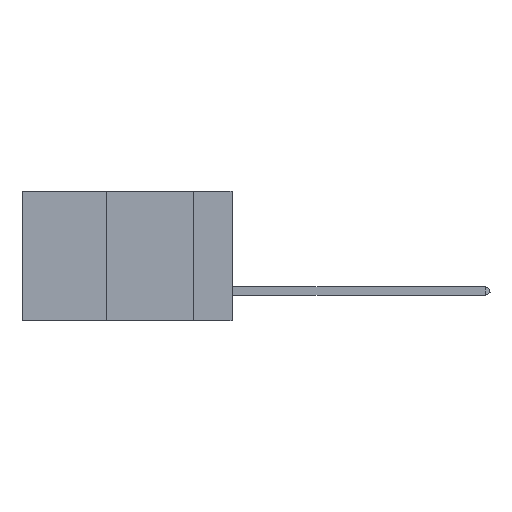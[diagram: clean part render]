
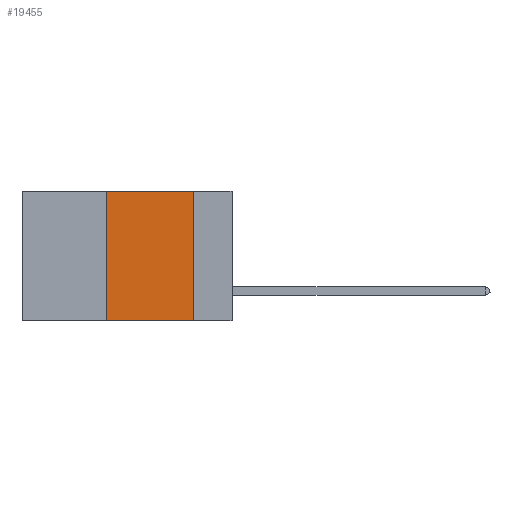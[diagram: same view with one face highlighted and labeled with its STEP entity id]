
A CAD part, left-side view. The second image highlights one B-rep face of the part: STEP entity #19455.
In plain terms, the highlighted planar face has unit normal (-1, 0, 0).
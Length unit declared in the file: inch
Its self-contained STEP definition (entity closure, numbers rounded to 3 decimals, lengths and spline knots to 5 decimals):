
#2512 = EDGE_LOOP ( 'NONE', ( #15538, #45953, #48157, #13108 ) ) ;
#3488 = LINE ( 'NONE', #41045, #7559 ) ;
#4142 = AXIS2_PLACEMENT_3D ( 'NONE', #28260, #43907, #5815 ) ;
#5815 = DIRECTION ( 'NONE',  ( 0., 0., -1. ) ) ;
#7559 = VECTOR ( 'NONE', #26187, 39.37008 ) ;
#9216 = CARTESIAN_POINT ( 'NONE',  ( 0., 0.6, -0.37 ) ) ;
#12147 = LINE ( 'NONE', #9216, #47156 ) ;
#13108 = ORIENTED_EDGE ( 'NONE', *, *, #34839, .T. ) ;
#13421 = DIRECTION ( 'NONE',  ( 0., -1., 0. ) ) ;
#14408 = VERTEX_POINT ( 'NONE', #39909 ) ;
#14784 = LINE ( 'NONE', #43651, #22432 ) ;
#15224 = VECTOR ( 'NONE', #18230, 39.37008 ) ;
#15538 = ORIENTED_EDGE ( 'NONE', *, *, #29078, .F. ) ;
#18230 = DIRECTION ( 'NONE',  ( 0., -1., 0. ) ) ;
#19455 = ADVANCED_FACE ( 'NONE', ( #45146 ), #36303, .F. ) ;
#21115 = CARTESIAN_POINT ( 'NONE',  ( 0., 0.36, 0. ) ) ;
#22432 = VECTOR ( 'NONE', #47634, 39.37008 ) ;
#22565 = EDGE_CURVE ( 'NONE', #42431, #14408, #34150, .T. ) ;
#25811 = CARTESIAN_POINT ( 'NONE',  ( 0., 0.36, -0.37 ) ) ;
#26187 = DIRECTION ( 'NONE',  ( 0., 0., 1. ) ) ;
#28260 = CARTESIAN_POINT ( 'NONE',  ( 0., 0.6, 0. ) ) ;
#29078 = EDGE_CURVE ( 'NONE', #14408, #37058, #14784, .T. ) ;
#29113 = CARTESIAN_POINT ( 'NONE',  ( 0., 0.11, -0.37 ) ) ;
#29294 = EDGE_CURVE ( 'NONE', #37405, #42431, #3488, .T. ) ;
#34150 = LINE ( 'NONE', #43219, #15224 ) ;
#34839 = EDGE_CURVE ( 'NONE', #37405, #37058, #12147, .T. ) ;
#36303 = PLANE ( 'NONE',  #4142 ) ;
#37058 = VERTEX_POINT ( 'NONE', #29113 ) ;
#37405 = VERTEX_POINT ( 'NONE', #25811 ) ;
#39909 = CARTESIAN_POINT ( 'NONE',  ( 0., 0.11, 0. ) ) ;
#41045 = CARTESIAN_POINT ( 'NONE',  ( 0., 0.36, 0. ) ) ;
#42431 = VERTEX_POINT ( 'NONE', #21115 ) ;
#43219 = CARTESIAN_POINT ( 'NONE',  ( 0., 0.6, 0. ) ) ;
#43651 = CARTESIAN_POINT ( 'NONE',  ( 0., 0.11, 0. ) ) ;
#43907 = DIRECTION ( 'NONE',  ( 1., 0., 0. ) ) ;
#45146 = FACE_OUTER_BOUND ( 'NONE', #2512, .T. ) ;
#45953 = ORIENTED_EDGE ( 'NONE', *, *, #22565, .F. ) ;
#47156 = VECTOR ( 'NONE', #13421, 39.37008 ) ;
#47634 = DIRECTION ( 'NONE',  ( 0., 0., -1. ) ) ;
#48157 = ORIENTED_EDGE ( 'NONE', *, *, #29294, .F. ) ;
